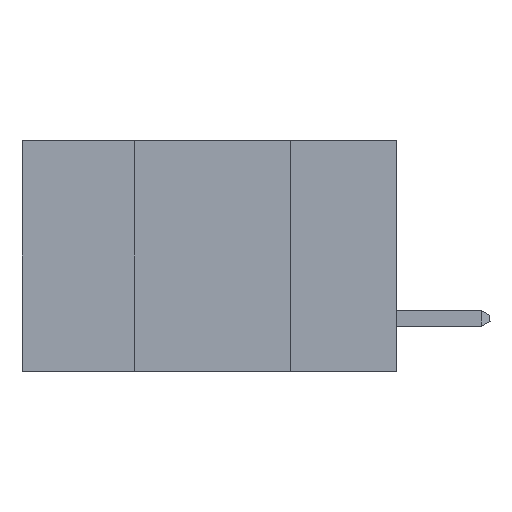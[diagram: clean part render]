
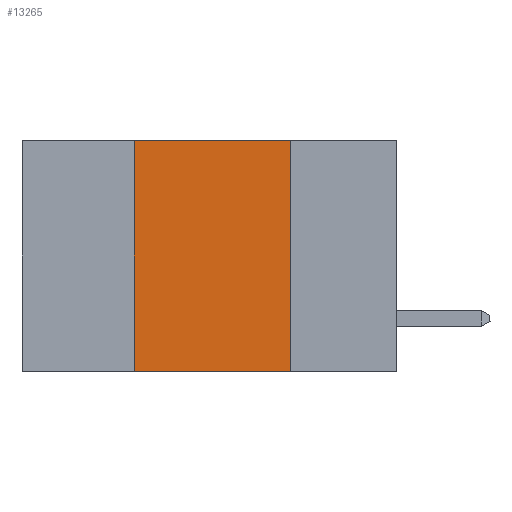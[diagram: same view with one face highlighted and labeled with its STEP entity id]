
A CAD part, left-side view. The second image highlights one B-rep face of the part: STEP entity #13265.
In plain terms, the highlighted planar face has unit normal (-1, 0, 0).
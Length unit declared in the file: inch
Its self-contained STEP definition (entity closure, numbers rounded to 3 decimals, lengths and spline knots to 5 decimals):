
#588 = DIRECTION ( 'NONE',  ( 0., 0., -1. ) ) ;
#1117 = LINE ( 'NONE', #10471, #5734 ) ;
#1416 = DIRECTION ( 'NONE',  ( 0., 0., -1. ) ) ;
#1721 = DIRECTION ( 'NONE',  ( 0., 0., 1. ) ) ;
#1806 = CARTESIAN_POINT ( 'NONE',  ( 0., 0.6, 0. ) ) ;
#3373 = VERTEX_POINT ( 'NONE', #13564 ) ;
#3726 = ORIENTED_EDGE ( 'NONE', *, *, #11533, .T. ) ;
#3959 = ORIENTED_EDGE ( 'NONE', *, *, #8762, .F. ) ;
#4673 = VERTEX_POINT ( 'NONE', #5797 ) ;
#4913 = LINE ( 'NONE', #1806, #11504 ) ;
#5648 = DIRECTION ( 'NONE',  ( 1., 0., 0. ) ) ;
#5734 = VECTOR ( 'NONE', #9431, 39.37008 ) ;
#5797 = CARTESIAN_POINT ( 'NONE',  ( 0., 0.42, 0. ) ) ;
#6088 = ORIENTED_EDGE ( 'NONE', *, *, #11158, .F. ) ;
#6563 = CARTESIAN_POINT ( 'NONE',  ( 0., 0.6, 0. ) ) ;
#6572 = EDGE_CURVE ( 'NONE', #11791, #3373, #9936, .T. ) ;
#6641 = VERTEX_POINT ( 'NONE', #10266 ) ;
#7917 = EDGE_LOOP ( 'NONE', ( #11474, #3959, #6088, #3726 ) ) ;
#7962 = CARTESIAN_POINT ( 'NONE',  ( 0., 0.42, 0. ) ) ;
#8762 = EDGE_CURVE ( 'NONE', #4673, #11791, #4913, .T. ) ;
#9088 = FACE_OUTER_BOUND ( 'NONE', #7917, .T. ) ;
#9431 = DIRECTION ( 'NONE',  ( 0., -1., 0. ) ) ;
#9763 = LINE ( 'NONE', #7962, #12570 ) ;
#9936 = LINE ( 'NONE', #11088, #11415 ) ;
#10266 = CARTESIAN_POINT ( 'NONE',  ( 0., 0.42, -0.37 ) ) ;
#10471 = CARTESIAN_POINT ( 'NONE',  ( 0., 0.6, -0.37 ) ) ;
#10817 = PLANE ( 'NONE',  #12845 ) ;
#11088 = CARTESIAN_POINT ( 'NONE',  ( 0., 0.17, 0. ) ) ;
#11158 = EDGE_CURVE ( 'NONE', #6641, #4673, #9763, .T. ) ;
#11415 = VECTOR ( 'NONE', #588, 39.37008 ) ;
#11474 = ORIENTED_EDGE ( 'NONE', *, *, #6572, .F. ) ;
#11504 = VECTOR ( 'NONE', #13453, 39.37008 ) ;
#11533 = EDGE_CURVE ( 'NONE', #6641, #3373, #1117, .T. ) ;
#11791 = VERTEX_POINT ( 'NONE', #13252 ) ;
#12570 = VECTOR ( 'NONE', #1721, 39.37008 ) ;
#12845 = AXIS2_PLACEMENT_3D ( 'NONE', #6563, #5648, #1416 ) ;
#13252 = CARTESIAN_POINT ( 'NONE',  ( 0., 0.17, 0. ) ) ;
#13265 = ADVANCED_FACE ( 'NONE', ( #9088 ), #10817, .F. ) ;
#13453 = DIRECTION ( 'NONE',  ( 0., -1., 0. ) ) ;
#13564 = CARTESIAN_POINT ( 'NONE',  ( 0., 0.17, -0.37 ) ) ;
